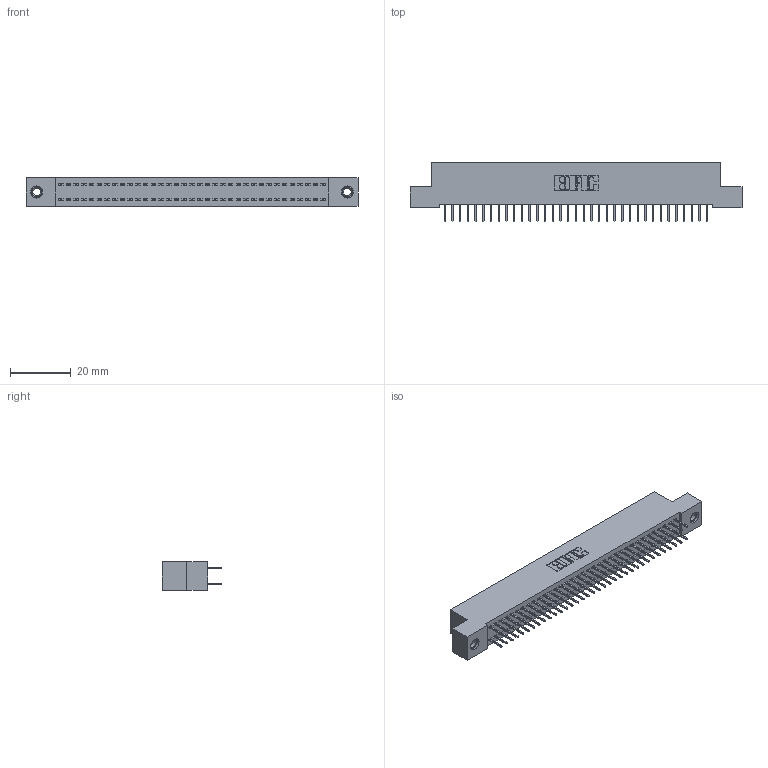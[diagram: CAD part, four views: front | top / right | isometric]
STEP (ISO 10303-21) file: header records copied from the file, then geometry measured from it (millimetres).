
FILE_DESCRIPTION (( 'STEP AP203' ), '1' );
FILE_NAME ('342-070-524-207.STEP', '2018-08-13T09:21:49', ( '' ), ( '' ), 'SwSTEP 2.0', 'SolidWorks 2016', '' );
FILE_SCHEMA (( 'CONFIG_CONTROL_DESIGN' ));
Length unit declared in the file: inch
Products named in the file (4): 342 Part_TI; 345-292-001_345-293-124; 345-250-001_345-250-005-103; 342-070-524-207
Assembly tree (73 placements, depth 2):
  342-070-524-207
    342 Part_TI
    345-292-001_345-293-124  x70
    345-250-001_345-250-005-103  x2
Bounding box: 109.22 x 19.69 x 9.4 mm (x, y, z)
Volume: 9661.7 mm3; surface area: 15304.5 mm2
Topology: 73 solids, 73 shells, 4090 faces, 11565 edges, 7422 vertices
Faces by surface type: plane 3038, cylinder 1036, cone 12, torus 4
Entity records: 24550 total; most frequent: CARTESIAN_POINT 4057, ORIENTED_EDGE 3986, DIRECTION 3511, EDGE_CURVE 1993, LINE 1849, VECTOR 1849, VERTEX_POINT 1320, AXIS2_PLACEMENT_3D 831
